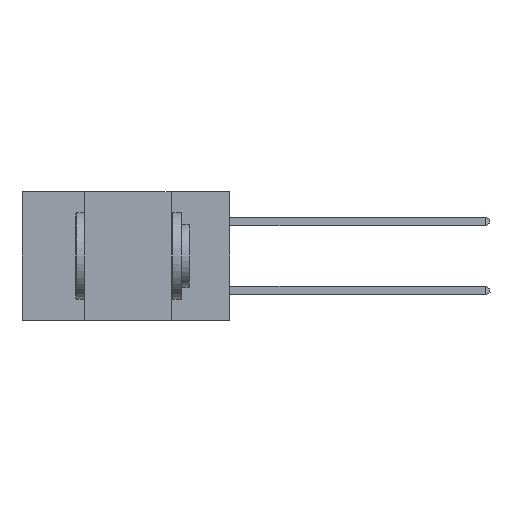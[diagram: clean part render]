
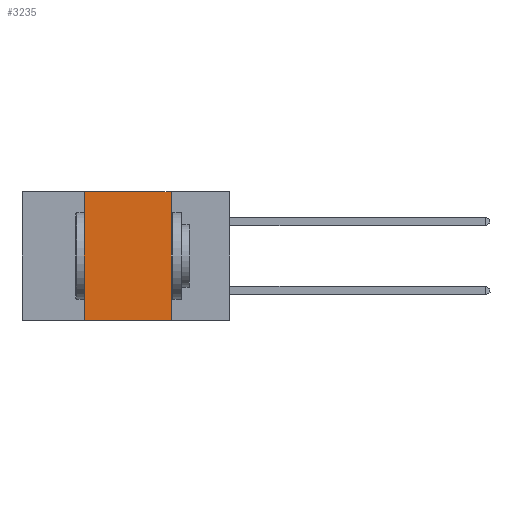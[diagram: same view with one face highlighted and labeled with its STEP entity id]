
A CAD part, left-side view. The second image highlights one B-rep face of the part: STEP entity #3235.
In plain terms, the highlighted planar face has unit normal (-1, 0, 0).
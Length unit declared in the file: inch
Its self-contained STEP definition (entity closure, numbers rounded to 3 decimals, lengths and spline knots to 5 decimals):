
#603 = EDGE_LOOP ( 'NONE', ( #5204, #17767, #2437, #22217 ) ) ;
#902 = LINE ( 'NONE', #4201, #19975 ) ;
#1344 = VECTOR ( 'NONE', #19256, 39.37008 ) ;
#1890 = VECTOR ( 'NONE', #17935, 39.37008 ) ;
#2031 = CARTESIAN_POINT ( 'NONE',  ( 0., 0.42, 0. ) ) ;
#2311 = DIRECTION ( 'NONE',  ( 0., -1., 0. ) ) ;
#2372 = FACE_OUTER_BOUND ( 'NONE', #603, .T. ) ;
#2437 = ORIENTED_EDGE ( 'NONE', *, *, #25354, .F. ) ;
#3235 = ADVANCED_FACE ( 'NONE', ( #2372 ), #17247, .F. ) ;
#3739 = DIRECTION ( 'NONE',  ( 0., 0., -1. ) ) ;
#4201 = CARTESIAN_POINT ( 'NONE',  ( 0., 0.6, -0.37 ) ) ;
#5204 = ORIENTED_EDGE ( 'NONE', *, *, #16620, .F. ) ;
#6035 = CARTESIAN_POINT ( 'NONE',  ( 0., 0.42, -0.37 ) ) ;
#7194 = LINE ( 'NONE', #23077, #1344 ) ;
#8055 = DIRECTION ( 'NONE',  ( 0., 0., 1. ) ) ;
#10127 = CARTESIAN_POINT ( 'NONE',  ( 0., 0.17, 0. ) ) ;
#11915 = EDGE_CURVE ( 'NONE', #23603, #21026, #7194, .T. ) ;
#12200 = VERTEX_POINT ( 'NONE', #24648 ) ;
#13375 = VERTEX_POINT ( 'NONE', #6035 ) ;
#13908 = LINE ( 'NONE', #2031, #16362 ) ;
#15457 = CARTESIAN_POINT ( 'NONE',  ( 0., 0.6, 0. ) ) ;
#15540 = DIRECTION ( 'NONE',  ( 1., 0., 0. ) ) ;
#16362 = VECTOR ( 'NONE', #8055, 39.37008 ) ;
#16620 = EDGE_CURVE ( 'NONE', #21026, #12200, #22781, .T. ) ;
#17247 = PLANE ( 'NONE',  #24499 ) ;
#17666 = CARTESIAN_POINT ( 'NONE',  ( 0., 0.17, 0. ) ) ;
#17767 = ORIENTED_EDGE ( 'NONE', *, *, #11915, .F. ) ;
#17935 = DIRECTION ( 'NONE',  ( 0., 0., -1. ) ) ;
#18142 = EDGE_CURVE ( 'NONE', #13375, #12200, #902, .T. ) ;
#19256 = DIRECTION ( 'NONE',  ( 0., -1., 0. ) ) ;
#19975 = VECTOR ( 'NONE', #2311, 39.37008 ) ;
#21026 = VERTEX_POINT ( 'NONE', #10127 ) ;
#22217 = ORIENTED_EDGE ( 'NONE', *, *, #18142, .T. ) ;
#22781 = LINE ( 'NONE', #17666, #1890 ) ;
#23077 = CARTESIAN_POINT ( 'NONE',  ( 0., 0.6, 0. ) ) ;
#23431 = CARTESIAN_POINT ( 'NONE',  ( 0., 0.42, 0. ) ) ;
#23603 = VERTEX_POINT ( 'NONE', #23431 ) ;
#24499 = AXIS2_PLACEMENT_3D ( 'NONE', #15457, #15540, #3739 ) ;
#24648 = CARTESIAN_POINT ( 'NONE',  ( 0., 0.17, -0.37 ) ) ;
#25354 = EDGE_CURVE ( 'NONE', #13375, #23603, #13908, .T. ) ;
